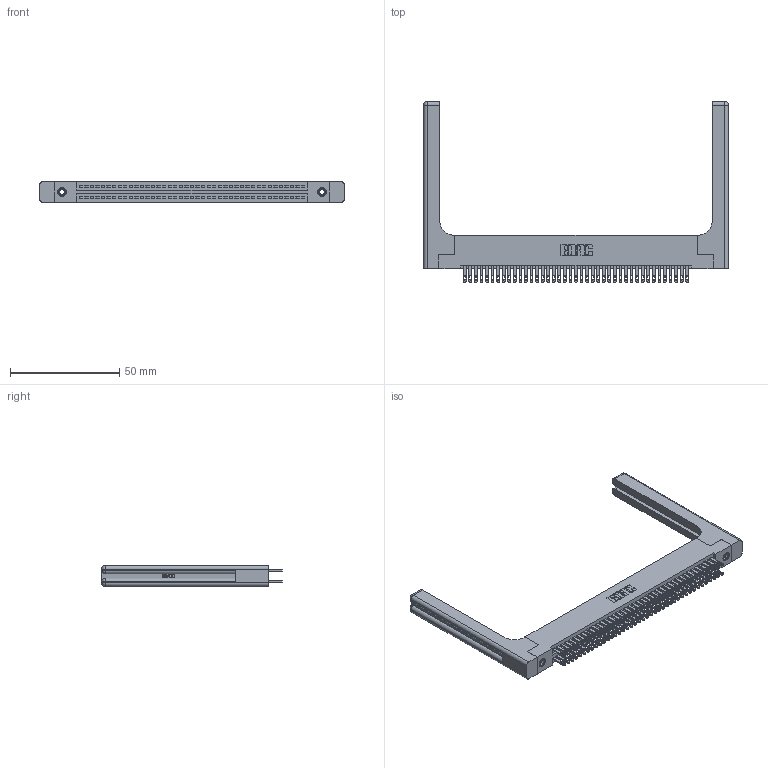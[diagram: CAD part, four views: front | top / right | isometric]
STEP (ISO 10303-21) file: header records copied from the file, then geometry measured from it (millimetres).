
FILE_DESCRIPTION (( 'STEP AP203' ), '1' );
FILE_NAME ('345-082-500-258.STEP', '2019-10-31T21:25:26', ( '' ), ( '' ), 'SwSTEP 2.0', 'SolidWorks 2016', '' );
FILE_SCHEMA (( 'CONFIG_CONTROL_DESIGN' ));
Length unit declared in the file: inch
Products named in the file (5): 345-292-001_345-293-100; 345-220-058_345-220-058; 345-082-500-258; 345 Part_Flush Mounting Lugs - 0.156 Dia-TH; 345-250-001_345-250-001-102
Assembly tree (87 placements, depth 2):
  345-082-500-258
    345 Part_Flush Mounting Lugs - 0.156 Dia-TH
    345-292-001_345-293-100  x82
    345-250-001_345-250-001-102  x2
    345-220-058_345-220-058  x2
Bounding box: 139.17 x 82.47 x 9.4 mm (x, y, z)
Volume: 22235.2 mm3; surface area: 26215.6 mm2
Topology: 87 solids, 87 shells, 4154 faces, 12569 edges, 8358 vertices
Faces by surface type: plane 2442, cylinder 1652, bspline 36, cone 12, sphere 8, torus 4
Entity records: 37416 total; most frequent: CARTESIAN_POINT 7265, ORIENTED_EDGE 5996, DIRECTION 5342, EDGE_CURVE 2998, LINE 2606, VECTOR 2606, VERTEX_POINT 1990, AXIS2_PLACEMENT_3D 1368
